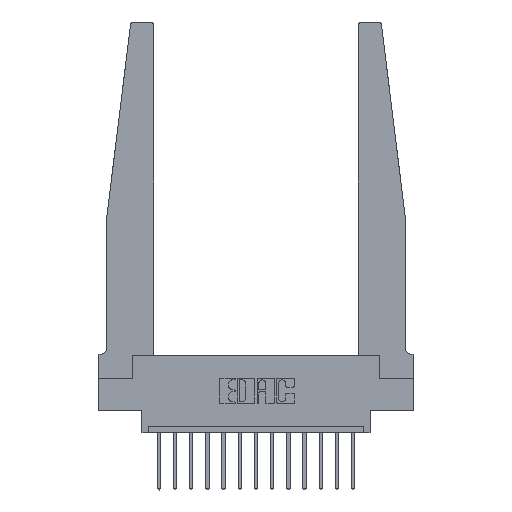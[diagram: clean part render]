
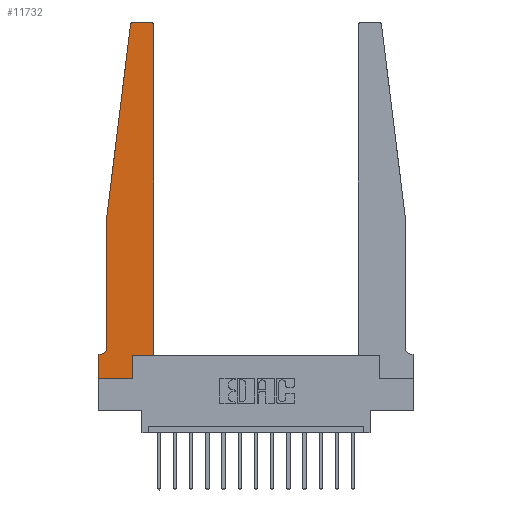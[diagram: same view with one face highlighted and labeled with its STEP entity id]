
A CAD part, top view. The second image highlights one B-rep face of the part: STEP entity #11732.
In plain terms, the highlighted planar face has unit normal (0, 0, 1).
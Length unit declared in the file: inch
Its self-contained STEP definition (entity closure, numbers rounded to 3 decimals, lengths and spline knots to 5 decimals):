
#65 = EDGE_CURVE ( 'NONE', #9151, #2782, #13870, .T. ) ;
#622 = VERTEX_POINT ( 'NONE', #10367 ) ;
#914 = VERTEX_POINT ( 'NONE', #6544 ) ;
#1238 = VERTEX_POINT ( 'NONE', #15069 ) ;
#1402 = CARTESIAN_POINT ( 'NONE',  ( 0.27653, 2.75, 0.37 ) ) ;
#1483 = EDGE_CURVE ( 'NONE', #7704, #16112, #16243, .T. ) ;
#1593 = EDGE_CURVE ( 'NONE', #1238, #7704, #3546, .T. ) ;
#1603 = CARTESIAN_POINT ( 'NONE',  ( 0.015, 0.2375, 0.37 ) ) ;
#1955 = CARTESIAN_POINT ( 'NONE',  ( 0.27653, 2.72, 0.37 ) ) ;
#2127 = LINE ( 'NONE', #11065, #11782 ) ;
#2328 = DIRECTION ( 'NONE',  ( 1., 0., 0. ) ) ;
#2582 = ORIENTED_EDGE ( 'NONE', *, *, #1593, .T. ) ;
#2596 = CARTESIAN_POINT ( 'NONE',  ( 0.425, 0.18, 0.37 ) ) ;
#2731 = EDGE_CURVE ( 'NONE', #914, #12717, #2127, .T. ) ;
#2782 = VERTEX_POINT ( 'NONE', #16052 ) ;
#2811 = VECTOR ( 'NONE', #15782, 39.37008 ) ;
#2965 = VECTOR ( 'NONE', #13894, 39.37008 ) ;
#3041 = EDGE_LOOP ( 'NONE', ( #15520, #12832, #10748, #15046, #11400, #16658, #9890, #2582, #10837, #5702, #5280, #6023 ) ) ;
#3546 = LINE ( 'NONE', #6151, #5194 ) ;
#3590 = LINE ( 'NONE', #4409, #5010 ) ;
#3653 = VECTOR ( 'NONE', #16219, 39.37008 ) ;
#3698 = VERTEX_POINT ( 'NONE', #5328 ) ;
#3808 = EDGE_CURVE ( 'NONE', #622, #15076, #14022, .T. ) ;
#4007 = CARTESIAN_POINT ( 'NONE',  ( 0.395, 2.72, 0.37 ) ) ;
#4378 = CARTESIAN_POINT ( 'NONE',  ( 0., 0., 0.37 ) ) ;
#4409 = CARTESIAN_POINT ( 'NONE',  ( 0.425, 0.18, 0.37 ) ) ;
#4584 = CARTESIAN_POINT ( 'NONE',  ( 0.065, 1.25, 0.37 ) ) ;
#4651 = FACE_OUTER_BOUND ( 'NONE', #3041, .T. ) ;
#4884 = LINE ( 'NONE', #4378, #3653 ) ;
#5010 = VECTOR ( 'NONE', #5865, 39.37008 ) ;
#5020 = DIRECTION ( 'NONE',  ( 1., 0., 0. ) ) ;
#5087 = CARTESIAN_POINT ( 'NONE',  ( 0., 0.1875, 0.37 ) ) ;
#5194 = VECTOR ( 'NONE', #2328, 39.37008 ) ;
#5280 = ORIENTED_EDGE ( 'NONE', *, *, #11697, .T. ) ;
#5328 = CARTESIAN_POINT ( 'NONE',  ( 0.065, 0.2375, 0.37 ) ) ;
#5378 = DIRECTION ( 'NONE',  ( 0., 0., 1. ) ) ;
#5681 = LINE ( 'NONE', #2596, #9611 ) ;
#5702 = ORIENTED_EDGE ( 'NONE', *, *, #13027, .T. ) ;
#5865 = DIRECTION ( 'NONE',  ( 1., 0., 0. ) ) ;
#5918 = DIRECTION ( 'NONE',  ( 0., -1., 0. ) ) ;
#6023 = ORIENTED_EDGE ( 'NONE', *, *, #14482, .T. ) ;
#6151 = CARTESIAN_POINT ( 'NONE',  ( 0., 0., 0.37 ) ) ;
#6460 = EDGE_CURVE ( 'NONE', #15076, #9151, #15083, .T. ) ;
#6544 = CARTESIAN_POINT ( 'NONE',  ( 0.015, 0.1875, 0.37 ) ) ;
#6658 = DIRECTION ( 'NONE',  ( 0., 0., 1. ) ) ;
#7249 = CARTESIAN_POINT ( 'NONE',  ( 0.425, 2.72, 0.37 ) ) ;
#7655 = AXIS2_PLACEMENT_3D ( 'NONE', #1955, #8540, #5020 ) ;
#7679 = PLANE ( 'NONE',  #15803 ) ;
#7704 = VERTEX_POINT ( 'NONE', #9400 ) ;
#7727 = AXIS2_PLACEMENT_3D ( 'NONE', #4007, #6658, #15799 ) ;
#8346 = CARTESIAN_POINT ( 'NONE',  ( 0.425, 0.18, 0.37 ) ) ;
#8468 = CIRCLE ( 'NONE', #7727, 0.03 ) ;
#8540 = DIRECTION ( 'NONE',  ( 0., 0., 1. ) ) ;
#8632 = CARTESIAN_POINT ( 'NONE',  ( 0.2605, 0.18, 0.37 ) ) ;
#9151 = VERTEX_POINT ( 'NONE', #14944 ) ;
#9400 = CARTESIAN_POINT ( 'NONE',  ( 0.2605, 0., 0.37 ) ) ;
#9529 = CARTESIAN_POINT ( 'NONE',  ( 0.2605, 0.18, 0.37 ) ) ;
#9611 = VECTOR ( 'NONE', #16899, 39.37008 ) ;
#9890 = ORIENTED_EDGE ( 'NONE', *, *, #11341, .T. ) ;
#10222 = VERTEX_POINT ( 'NONE', #7249 ) ;
#10367 = CARTESIAN_POINT ( 'NONE',  ( 0.395, 2.75, 0.37 ) ) ;
#10381 = AXIS2_PLACEMENT_3D ( 'NONE', #1603, #10988, #16062 ) ;
#10617 = CIRCLE ( 'NONE', #10381, 0.05 ) ;
#10717 = VERTEX_POINT ( 'NONE', #8346 ) ;
#10748 = ORIENTED_EDGE ( 'NONE', *, *, #65, .T. ) ;
#10837 = ORIENTED_EDGE ( 'NONE', *, *, #1483, .T. ) ;
#10988 = DIRECTION ( 'NONE',  ( 0., 0., -1. ) ) ;
#11065 = CARTESIAN_POINT ( 'NONE',  ( 0.065, 0.1875, 0.37 ) ) ;
#11341 = EDGE_CURVE ( 'NONE', #12717, #1238, #4884, .T. ) ;
#11370 = DIRECTION ( 'NONE',  ( -1., 0., 0. ) ) ;
#11400 = ORIENTED_EDGE ( 'NONE', *, *, #12496, .T. ) ;
#11697 = EDGE_CURVE ( 'NONE', #10717, #10222, #5681, .T. ) ;
#11732 = ADVANCED_FACE ( 'NONE', ( #4651 ), #7679, .T. ) ;
#11782 = VECTOR ( 'NONE', #16238, 39.37008 ) ;
#11909 = DIRECTION ( 'NONE',  ( 1., 0., 0. ) ) ;
#12496 = EDGE_CURVE ( 'NONE', #3698, #914, #10617, .T. ) ;
#12606 = CARTESIAN_POINT ( 'NONE',  ( 0.065, 1.25, 0.37 ) ) ;
#12717 = VERTEX_POINT ( 'NONE', #5087 ) ;
#12832 = ORIENTED_EDGE ( 'NONE', *, *, #6460, .T. ) ;
#12936 = LINE ( 'NONE', #4584, #15388 ) ;
#13027 = EDGE_CURVE ( 'NONE', #16112, #10717, #3590, .T. ) ;
#13595 = VECTOR ( 'NONE', #11370, 39.37008 ) ;
#13870 = LINE ( 'NONE', #12606, #2811 ) ;
#13894 = DIRECTION ( 'NONE',  ( 0., 1., 0. ) ) ;
#14022 = LINE ( 'NONE', #15530, #13595 ) ;
#14482 = EDGE_CURVE ( 'NONE', #10222, #622, #8468, .T. ) ;
#14944 = CARTESIAN_POINT ( 'NONE',  ( 0.24675, 2.72367, 0.37 ) ) ;
#15046 = ORIENTED_EDGE ( 'NONE', *, *, #15574, .T. ) ;
#15069 = CARTESIAN_POINT ( 'NONE',  ( 0., 0., 0.37 ) ) ;
#15076 = VERTEX_POINT ( 'NONE', #1402 ) ;
#15083 = CIRCLE ( 'NONE', #7655, 0.03 ) ;
#15388 = VECTOR ( 'NONE', #5918, 39.37008 ) ;
#15520 = ORIENTED_EDGE ( 'NONE', *, *, #3808, .T. ) ;
#15530 = CARTESIAN_POINT ( 'NONE',  ( 0.25, 2.75, 0.37 ) ) ;
#15574 = EDGE_CURVE ( 'NONE', #2782, #3698, #12936, .T. ) ;
#15782 = DIRECTION ( 'NONE',  ( -0.122, -0.992, 0. ) ) ;
#15799 = DIRECTION ( 'NONE',  ( 1., 0., 0. ) ) ;
#15803 = AXIS2_PLACEMENT_3D ( 'NONE', #15901, #5378, #11909 ) ;
#15901 = CARTESIAN_POINT ( 'NONE',  ( 0., 0.1875, 0.37 ) ) ;
#16052 = CARTESIAN_POINT ( 'NONE',  ( 0.065, 1.25, 0.37 ) ) ;
#16062 = DIRECTION ( 'NONE',  ( -1., 0., 0. ) ) ;
#16112 = VERTEX_POINT ( 'NONE', #9529 ) ;
#16219 = DIRECTION ( 'NONE',  ( 0., -1., 0. ) ) ;
#16238 = DIRECTION ( 'NONE',  ( -1., 0., 0. ) ) ;
#16243 = LINE ( 'NONE', #8632, #2965 ) ;
#16658 = ORIENTED_EDGE ( 'NONE', *, *, #2731, .T. ) ;
#16899 = DIRECTION ( 'NONE',  ( 0., 1., 0. ) ) ;
